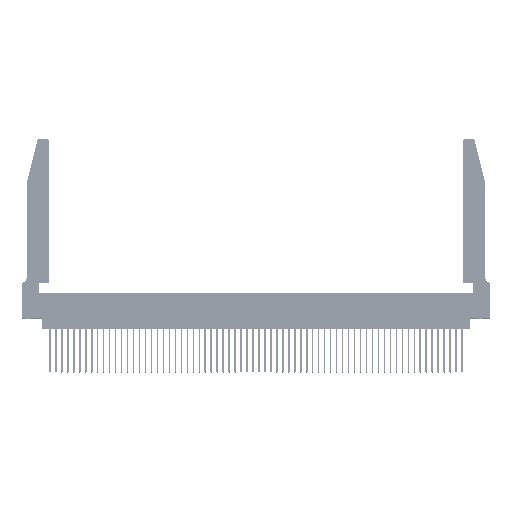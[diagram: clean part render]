
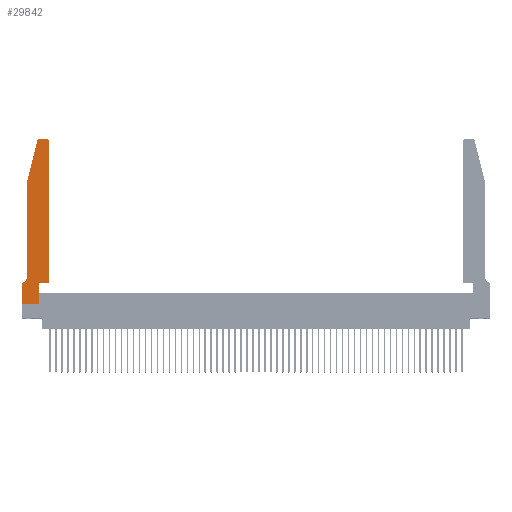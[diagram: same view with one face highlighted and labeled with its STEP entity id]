
A CAD part, top view. The second image highlights one B-rep face of the part: STEP entity #29842.
In plain terms, the highlighted planar face has unit normal (0, 0, 1).
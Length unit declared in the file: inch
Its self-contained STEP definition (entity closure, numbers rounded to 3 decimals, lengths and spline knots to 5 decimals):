
#826 = EDGE_CURVE ( 'NONE', #8214, #45529, #46884, .T. ) ;
#1440 = VERTEX_POINT ( 'NONE', #55443 ) ;
#1458 = CARTESIAN_POINT ( 'NONE',  ( 0.284, 2.75, 0.37 ) ) ;
#2351 = DIRECTION ( 'NONE',  ( 0., -1., 0. ) ) ;
#3081 = VERTEX_POINT ( 'NONE', #53369 ) ;
#3172 = LINE ( 'NONE', #22850, #28246 ) ;
#3199 = DIRECTION ( 'NONE',  ( 0., 0., 1. ) ) ;
#3220 = ORIENTED_EDGE ( 'NONE', *, *, #8359, .T. ) ;
#3247 = ORIENTED_EDGE ( 'NONE', *, *, #22281, .T. ) ;
#3823 = CARTESIAN_POINT ( 'NONE',  ( 0.4205, 2.72, 0.37 ) ) ;
#4502 = DIRECTION ( 'NONE',  ( 1., 0., 0. ) ) ;
#5003 = AXIS2_PLACEMENT_3D ( 'NONE', #51457, #3199, #50908 ) ;
#6894 = EDGE_LOOP ( 'NONE', ( #22418, #3247, #47259, #48962, #39708, #47397, #3220, #34021, #11797, #34209, #38227, #24736 ) ) ;
#7072 = FACE_OUTER_BOUND ( 'NONE', #6894, .T. ) ;
#8152 = DIRECTION ( 'NONE',  ( 0., 0., 1. ) ) ;
#8214 = VERTEX_POINT ( 'NONE', #35104 ) ;
#8359 = EDGE_CURVE ( 'NONE', #3081, #13867, #31162, .T. ) ;
#9740 = CARTESIAN_POINT ( 'NONE',  ( 0.4505, 0.35, 0.37 ) ) ;
#9766 = VECTOR ( 'NONE', #36891, 39.37008 ) ;
#11027 = VECTOR ( 'NONE', #45619, 39.37008 ) ;
#11797 = ORIENTED_EDGE ( 'NONE', *, *, #826, .T. ) ;
#11960 = CARTESIAN_POINT ( 'NONE',  ( 0.2865, 0.35, 0.37 ) ) ;
#12472 = CARTESIAN_POINT ( 'NONE',  ( 0.0055, 0.42, 0.37 ) ) ;
#13179 = CARTESIAN_POINT ( 'NONE',  ( 0., 0., 0.37 ) ) ;
#13464 = DIRECTION ( 'NONE',  ( 1., 0., 0. ) ) ;
#13849 = CARTESIAN_POINT ( 'NONE',  ( 0.284, 2.72, 0.37 ) ) ;
#13867 = VERTEX_POINT ( 'NONE', #44559 ) ;
#14033 = DIRECTION ( 'NONE',  ( 0., 0., 1. ) ) ;
#14592 = CARTESIAN_POINT ( 'NONE',  ( 0.0755, 0.42, 0.37 ) ) ;
#15638 = EDGE_CURVE ( 'NONE', #13867, #8214, #55741, .T. ) ;
#15909 = EDGE_CURVE ( 'NONE', #45529, #42390, #41538, .T. ) ;
#16741 = EDGE_CURVE ( 'NONE', #26109, #33109, #38756, .T. ) ;
#16875 = DIRECTION ( 'NONE',  ( 1., 0., 0. ) ) ;
#17552 = VERTEX_POINT ( 'NONE', #1458 ) ;
#17674 = EDGE_CURVE ( 'NONE', #1440, #17552, #47719, .T. ) ;
#17963 = CARTESIAN_POINT ( 'NONE',  ( 0.0055, 0.35, 0.37 ) ) ;
#18480 = VECTOR ( 'NONE', #4502, 39.37008 ) ;
#19206 = EDGE_CURVE ( 'NONE', #26147, #1440, #28297, .T. ) ;
#19593 = LINE ( 'NONE', #47241, #52772 ) ;
#21709 = VERTEX_POINT ( 'NONE', #39268 ) ;
#22281 = EDGE_CURVE ( 'NONE', #17552, #21709, #49034, .T. ) ;
#22418 = ORIENTED_EDGE ( 'NONE', *, *, #17674, .T. ) ;
#22850 = CARTESIAN_POINT ( 'NONE',  ( 0.0755, 0.35, 0.37 ) ) ;
#23236 = CARTESIAN_POINT ( 'NONE',  ( 0.0755, 2., 0.37 ) ) ;
#24736 = ORIENTED_EDGE ( 'NONE', *, *, #19206, .T. ) ;
#26109 = VERTEX_POINT ( 'NONE', #23236 ) ;
#26147 = VERTEX_POINT ( 'NONE', #44484 ) ;
#26352 = CARTESIAN_POINT ( 'NONE',  ( 0.0755, 2., 0.37 ) ) ;
#26428 = VECTOR ( 'NONE', #2351, 39.37008 ) ;
#26510 = EDGE_CURVE ( 'NONE', #42390, #26147, #30524, .T. ) ;
#28246 = VECTOR ( 'NONE', #53899, 39.37008 ) ;
#28297 = CIRCLE ( 'NONE', #40275, 0.03 ) ;
#29842 = ADVANCED_FACE ( 'NONE', ( #7072 ), #42235, .T. ) ;
#30524 = LINE ( 'NONE', #55194, #41370 ) ;
#31162 = LINE ( 'NONE', #32079, #26428 ) ;
#32079 = CARTESIAN_POINT ( 'NONE',  ( 0., 0., 0.37 ) ) ;
#32736 = CIRCLE ( 'NONE', #55797, 0.07 ) ;
#33109 = VERTEX_POINT ( 'NONE', #14592 ) ;
#33632 = DIRECTION ( 'NONE',  ( 0., 1., 0. ) ) ;
#34021 = ORIENTED_EDGE ( 'NONE', *, *, #15638, .T. ) ;
#34167 = DIRECTION ( 'NONE',  ( -0.239, -0.971, 0. ) ) ;
#34209 = ORIENTED_EDGE ( 'NONE', *, *, #15909, .T. ) ;
#34503 = DIRECTION ( 'NONE',  ( 0., -1., 0. ) ) ;
#35104 = CARTESIAN_POINT ( 'NONE',  ( 0.2865, 0., 0.37 ) ) ;
#36313 = CARTESIAN_POINT ( 'NONE',  ( 0.2605, 2.75, 0.37 ) ) ;
#36877 = CARTESIAN_POINT ( 'NONE',  ( 0.4505, 0.35, 0.37 ) ) ;
#36891 = DIRECTION ( 'NONE',  ( -1., 0., 0. ) ) ;
#38065 = VECTOR ( 'NONE', #54779, 39.37008 ) ;
#38227 = ORIENTED_EDGE ( 'NONE', *, *, #26510, .T. ) ;
#38257 = DIRECTION ( 'NONE',  ( -1., 0., 0. ) ) ;
#38756 = LINE ( 'NONE', #26352, #41504 ) ;
#39268 = CARTESIAN_POINT ( 'NONE',  ( 0.25487, 2.72718, 0.37 ) ) ;
#39708 = ORIENTED_EDGE ( 'NONE', *, *, #54123, .T. ) ;
#40275 = AXIS2_PLACEMENT_3D ( 'NONE', #3823, #8152, #16875 ) ;
#41370 = VECTOR ( 'NONE', #33632, 39.37008 ) ;
#41504 = VECTOR ( 'NONE', #34503, 39.37008 ) ;
#41538 = LINE ( 'NONE', #36877, #11027 ) ;
#42235 = PLANE ( 'NONE',  #5003 ) ;
#42390 = VERTEX_POINT ( 'NONE', #9740 ) ;
#43720 = EDGE_CURVE ( 'NONE', #50543, #3081, #3172, .T. ) ;
#44484 = CARTESIAN_POINT ( 'NONE',  ( 0.4505, 2.72, 0.37 ) ) ;
#44559 = CARTESIAN_POINT ( 'NONE',  ( 0., 0., 0.37 ) ) ;
#45451 = AXIS2_PLACEMENT_3D ( 'NONE', #13849, #14033, #13464 ) ;
#45529 = VERTEX_POINT ( 'NONE', #50396 ) ;
#45619 = DIRECTION ( 'NONE',  ( 1., 0., 0. ) ) ;
#46884 = LINE ( 'NONE', #11960, #38065 ) ;
#47241 = CARTESIAN_POINT ( 'NONE',  ( 0.0755, 2., 0.37 ) ) ;
#47259 = ORIENTED_EDGE ( 'NONE', *, *, #49030, .T. ) ;
#47397 = ORIENTED_EDGE ( 'NONE', *, *, #43720, .T. ) ;
#47719 = LINE ( 'NONE', #36313, #9766 ) ;
#48962 = ORIENTED_EDGE ( 'NONE', *, *, #16741, .T. ) ;
#49030 = EDGE_CURVE ( 'NONE', #21709, #26109, #19593, .T. ) ;
#49034 = CIRCLE ( 'NONE', #45451, 0.03 ) ;
#50396 = CARTESIAN_POINT ( 'NONE',  ( 0.2865, 0.35, 0.37 ) ) ;
#50543 = VERTEX_POINT ( 'NONE', #17963 ) ;
#50908 = DIRECTION ( 'NONE',  ( 1., 0., 0. ) ) ;
#51457 = CARTESIAN_POINT ( 'NONE',  ( 0., 0.35, 0.37 ) ) ;
#51495 = DIRECTION ( 'NONE',  ( 0., 0., -1. ) ) ;
#52772 = VECTOR ( 'NONE', #34167, 39.37008 ) ;
#53369 = CARTESIAN_POINT ( 'NONE',  ( 0., 0.35, 0.37 ) ) ;
#53899 = DIRECTION ( 'NONE',  ( -1., 0., 0. ) ) ;
#54123 = EDGE_CURVE ( 'NONE', #33109, #50543, #32736, .T. ) ;
#54779 = DIRECTION ( 'NONE',  ( 0., 1., 0. ) ) ;
#55194 = CARTESIAN_POINT ( 'NONE',  ( 0.4505, 0.35, 0.37 ) ) ;
#55443 = CARTESIAN_POINT ( 'NONE',  ( 0.4205, 2.75, 0.37 ) ) ;
#55741 = LINE ( 'NONE', #13179, #18480 ) ;
#55797 = AXIS2_PLACEMENT_3D ( 'NONE', #12472, #51495, #38257 ) ;
